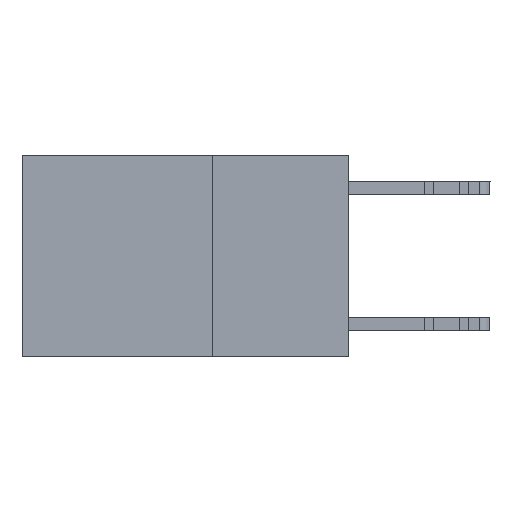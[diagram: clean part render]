
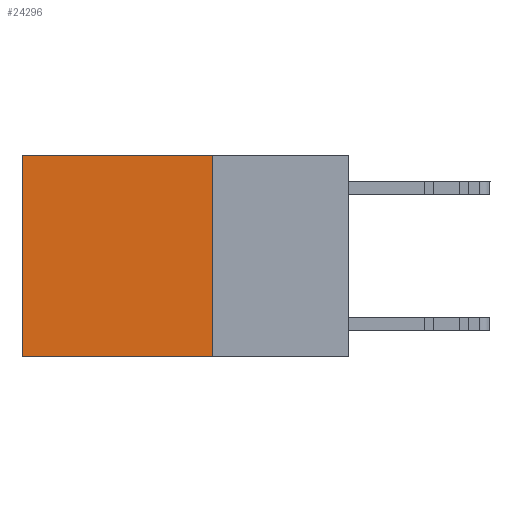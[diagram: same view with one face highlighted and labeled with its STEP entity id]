
A CAD part, left-side view. The second image highlights one B-rep face of the part: STEP entity #24296.
In plain terms, the highlighted planar face has unit normal (-1, 0, 0).
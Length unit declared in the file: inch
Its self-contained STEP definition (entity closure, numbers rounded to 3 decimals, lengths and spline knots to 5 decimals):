
#1648 = EDGE_CURVE ( 'NONE', #12374, #21459, #31559, .T. ) ;
#1947 = ORIENTED_EDGE ( 'NONE', *, *, #14267, .F. ) ;
#4709 = AXIS2_PLACEMENT_3D ( 'NONE', #13556, #23163, #25897 ) ;
#4813 = EDGE_CURVE ( 'NONE', #26649, #10594, #5451, .T. ) ;
#5451 = LINE ( 'NONE', #15251, #27588 ) ;
#6110 = ORIENTED_EDGE ( 'NONE', *, *, #25756, .T. ) ;
#9065 = DIRECTION ( 'NONE',  ( 0., 1., 0. ) ) ;
#9260 = DIRECTION ( 'NONE',  ( 0., 0., -1. ) ) ;
#10594 = VERTEX_POINT ( 'NONE', #18940 ) ;
#12374 = VERTEX_POINT ( 'NONE', #27593 ) ;
#13556 = CARTESIAN_POINT ( 'NONE',  ( 0.2625, 0.25, 0. ) ) ;
#13608 = CARTESIAN_POINT ( 'NONE',  ( 0.2625, 0.25, -0.37 ) ) ;
#14050 = LINE ( 'NONE', #30395, #19115 ) ;
#14199 = CARTESIAN_POINT ( 'NONE',  ( 0.2625, 0.25, -0.37 ) ) ;
#14267 = EDGE_CURVE ( 'NONE', #21459, #10594, #25622, .T. ) ;
#14296 = ORIENTED_EDGE ( 'NONE', *, *, #1648, .F. ) ;
#15192 = EDGE_LOOP ( 'NONE', ( #23899, #1947, #14296, #6110 ) ) ;
#15251 = CARTESIAN_POINT ( 'NONE',  ( 0.2625, 0.6, 0. ) ) ;
#16118 = FACE_OUTER_BOUND ( 'NONE', #15192, .T. ) ;
#17486 = DIRECTION ( 'NONE',  ( 0., 0., -1. ) ) ;
#18144 = CARTESIAN_POINT ( 'NONE',  ( 0.2625, 0.6, 0. ) ) ;
#18940 = CARTESIAN_POINT ( 'NONE',  ( 0.2625, 0.6, -0.37 ) ) ;
#19115 = VECTOR ( 'NONE', #9065, 39.37008 ) ;
#19772 = VECTOR ( 'NONE', #23211, 39.37008 ) ;
#21296 = CARTESIAN_POINT ( 'NONE',  ( 0.2625, 0.25, 0. ) ) ;
#21459 = VERTEX_POINT ( 'NONE', #14199 ) ;
#23163 = DIRECTION ( 'NONE',  ( 1., 0., 0. ) ) ;
#23211 = DIRECTION ( 'NONE',  ( 0., 1., 0. ) ) ;
#23899 = ORIENTED_EDGE ( 'NONE', *, *, #4813, .T. ) ;
#24296 = ADVANCED_FACE ( 'NONE', ( #16118 ), #28465, .F. ) ;
#25254 = VECTOR ( 'NONE', #9260, 39.37008 ) ;
#25622 = LINE ( 'NONE', #13608, #19772 ) ;
#25756 = EDGE_CURVE ( 'NONE', #12374, #26649, #14050, .T. ) ;
#25897 = DIRECTION ( 'NONE',  ( 0., 0., -1. ) ) ;
#26649 = VERTEX_POINT ( 'NONE', #18144 ) ;
#27588 = VECTOR ( 'NONE', #17486, 39.37008 ) ;
#27593 = CARTESIAN_POINT ( 'NONE',  ( 0.2625, 0.25, 0. ) ) ;
#28465 = PLANE ( 'NONE',  #4709 ) ;
#30395 = CARTESIAN_POINT ( 'NONE',  ( 0.2625, 0.25, 0. ) ) ;
#31559 = LINE ( 'NONE', #21296, #25254 ) ;
